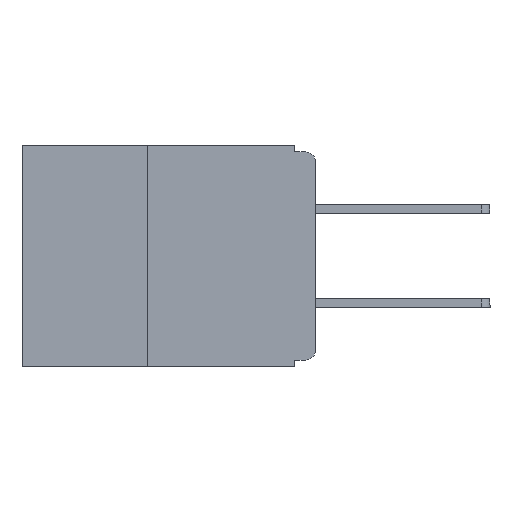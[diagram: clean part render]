
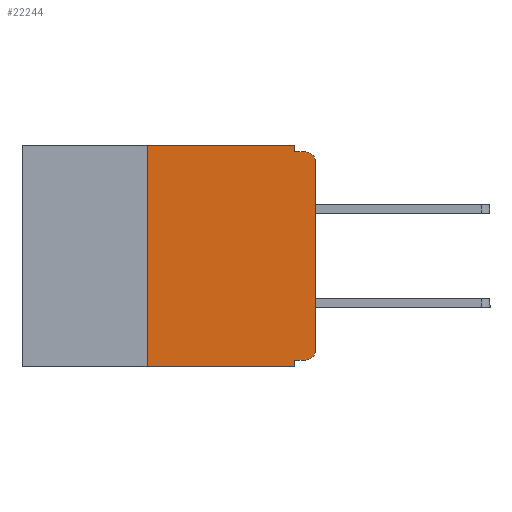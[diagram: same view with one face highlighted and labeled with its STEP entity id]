
A CAD part, left-side view. The second image highlights one B-rep face of the part: STEP entity #22244.
In plain terms, the highlighted planar face has unit normal (-1, 0, 0).
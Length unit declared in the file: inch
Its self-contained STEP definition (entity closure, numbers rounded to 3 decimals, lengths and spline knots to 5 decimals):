
#29 = EDGE_CURVE ( 'NONE', #1006, #13950, #11299, .T. ) ;
#1006 = VERTEX_POINT ( 'NONE', #7758 ) ;
#1195 = VECTOR ( 'NONE', #1696, 39.37008 ) ;
#1295 = CARTESIAN_POINT ( 'NONE',  ( 0., 0.437, 0. ) ) ;
#1696 = DIRECTION ( 'NONE',  ( 0., 1., 0. ) ) ;
#1912 = VERTEX_POINT ( 'NONE', #15409 ) ;
#1956 = ORIENTED_EDGE ( 'NONE', *, *, #19438, .T. ) ;
#3375 = AXIS2_PLACEMENT_3D ( 'NONE', #20729, #7607, #22904 ) ;
#3509 = VECTOR ( 'NONE', #16012, 39.37008 ) ;
#5172 = VECTOR ( 'NONE', #18934, 39.37008 ) ;
#5415 = VERTEX_POINT ( 'NONE', #25262 ) ;
#5727 = VERTEX_POINT ( 'NONE', #28318 ) ;
#6195 = ORIENTED_EDGE ( 'NONE', *, *, #29, .F. ) ;
#6895 = CARTESIAN_POINT ( 'NONE',  ( 0., 0.031, -0.33 ) ) ;
#6993 = VECTOR ( 'NONE', #25163, 39.37008 ) ;
#7089 = CARTESIAN_POINT ( 'NONE',  ( 0., 0.437, -0.33 ) ) ;
#7285 = CARTESIAN_POINT ( 'NONE',  ( 0., 0., -0.01 ) ) ;
#7607 = DIRECTION ( 'NONE',  ( -1., 0., 0. ) ) ;
#7673 = EDGE_CURVE ( 'NONE', #13950, #8500, #27749, .T. ) ;
#7758 = CARTESIAN_POINT ( 'NONE',  ( 0., 0.031, 0. ) ) ;
#7817 = CARTESIAN_POINT ( 'NONE',  ( 0., 0.015, -0.01 ) ) ;
#8166 = ORIENTED_EDGE ( 'NONE', *, *, #11229, .T. ) ;
#8500 = VERTEX_POINT ( 'NONE', #7817 ) ;
#8838 = VERTEX_POINT ( 'NONE', #8943 ) ;
#8943 = CARTESIAN_POINT ( 'NONE',  ( 0., 0., -0.025 ) ) ;
#9079 = ORIENTED_EDGE ( 'NONE', *, *, #23226, .T. ) ;
#9568 = ORIENTED_EDGE ( 'NONE', *, *, #26012, .F. ) ;
#10179 = CARTESIAN_POINT ( 'NONE',  ( 0., 0., 0. ) ) ;
#10299 = DIRECTION ( 'NONE',  ( 0., 0., -1. ) ) ;
#10563 = CIRCLE ( 'NONE', #24649, 0.015 ) ;
#10622 = VECTOR ( 'NONE', #17894, 39.37008 ) ;
#10719 = LINE ( 'NONE', #7089, #16551 ) ;
#11229 = EDGE_CURVE ( 'NONE', #1912, #5415, #12708, .T. ) ;
#11299 = LINE ( 'NONE', #25956, #10622 ) ;
#11710 = CARTESIAN_POINT ( 'NONE',  ( 0., 0.25, -0.33 ) ) ;
#12235 = ORIENTED_EDGE ( 'NONE', *, *, #26722, .F. ) ;
#12324 = CARTESIAN_POINT ( 'NONE',  ( 0., 0.015, -0.025 ) ) ;
#12623 = EDGE_CURVE ( 'NONE', #8838, #8500, #10563, .T. ) ;
#12708 = CIRCLE ( 'NONE', #3375, 0.015 ) ;
#12753 = EDGE_CURVE ( 'NONE', #1912, #5727, #12961, .T. ) ;
#12961 = LINE ( 'NONE', #17100, #1195 ) ;
#13812 = CARTESIAN_POINT ( 'NONE',  ( 0., 0.437, 0. ) ) ;
#13950 = VERTEX_POINT ( 'NONE', #21244 ) ;
#14534 = DIRECTION ( 'NONE',  ( 0., 0., -1. ) ) ;
#14730 = LINE ( 'NONE', #10179, #26298 ) ;
#14974 = EDGE_LOOP ( 'NONE', ( #1956, #27869, #20417, #6195, #9568, #12235, #9079, #20071, #25366, #8166 ) ) ;
#15409 = CARTESIAN_POINT ( 'NONE',  ( 0., 0.015, -0.32 ) ) ;
#16012 = DIRECTION ( 'NONE',  ( 0., -1., 0. ) ) ;
#16551 = VECTOR ( 'NONE', #20289, 39.37008 ) ;
#16734 = CARTESIAN_POINT ( 'NONE',  ( 0., 0.25, -0.33 ) ) ;
#16807 = PLANE ( 'NONE',  #22820 ) ;
#17100 = CARTESIAN_POINT ( 'NONE',  ( 0., 0., -0.32 ) ) ;
#17527 = LINE ( 'NONE', #16734, #5172 ) ;
#17894 = DIRECTION ( 'NONE',  ( 0., 0., -1. ) ) ;
#18116 = DIRECTION ( 'NONE',  ( 0., -1., 0. ) ) ;
#18645 = LINE ( 'NONE', #22978, #6993 ) ;
#18934 = DIRECTION ( 'NONE',  ( 0., 0., 1. ) ) ;
#19438 = EDGE_CURVE ( 'NONE', #5415, #8838, #14730, .T. ) ;
#20071 = ORIENTED_EDGE ( 'NONE', *, *, #22750, .F. ) ;
#20289 = DIRECTION ( 'NONE',  ( 0., -1., 0. ) ) ;
#20417 = ORIENTED_EDGE ( 'NONE', *, *, #7673, .F. ) ;
#20726 = FACE_OUTER_BOUND ( 'NONE', #14974, .T. ) ;
#20729 = CARTESIAN_POINT ( 'NONE',  ( 0., 0.015, -0.305 ) ) ;
#21001 = LINE ( 'NONE', #13812, #3509 ) ;
#21175 = VERTEX_POINT ( 'NONE', #11710 ) ;
#21244 = CARTESIAN_POINT ( 'NONE',  ( 0., 0.031, -0.01 ) ) ;
#21419 = VECTOR ( 'NONE', #18116, 39.37008 ) ;
#22244 = ADVANCED_FACE ( 'NONE', ( #20726 ), #16807, .F. ) ;
#22750 = EDGE_CURVE ( 'NONE', #5727, #26431, #18645, .T. ) ;
#22820 = AXIS2_PLACEMENT_3D ( 'NONE', #1295, #23378, #10299 ) ;
#22904 = DIRECTION ( 'NONE',  ( 0., 0., -1. ) ) ;
#22978 = CARTESIAN_POINT ( 'NONE',  ( 0., 0.031, -0.33 ) ) ;
#23226 = EDGE_CURVE ( 'NONE', #21175, #26431, #10719, .T. ) ;
#23378 = DIRECTION ( 'NONE',  ( 1., 0., 0. ) ) ;
#23645 = VERTEX_POINT ( 'NONE', #27912 ) ;
#24649 = AXIS2_PLACEMENT_3D ( 'NONE', #12324, #27471, #14534 ) ;
#25163 = DIRECTION ( 'NONE',  ( 0., 0., -1. ) ) ;
#25262 = CARTESIAN_POINT ( 'NONE',  ( 0., 0., -0.305 ) ) ;
#25366 = ORIENTED_EDGE ( 'NONE', *, *, #12753, .F. ) ;
#25956 = CARTESIAN_POINT ( 'NONE',  ( 0., 0.031, 0. ) ) ;
#26012 = EDGE_CURVE ( 'NONE', #23645, #1006, #21001, .T. ) ;
#26298 = VECTOR ( 'NONE', #27438, 39.37008 ) ;
#26431 = VERTEX_POINT ( 'NONE', #6895 ) ;
#26722 = EDGE_CURVE ( 'NONE', #21175, #23645, #17527, .T. ) ;
#27438 = DIRECTION ( 'NONE',  ( 0., 0., 1. ) ) ;
#27471 = DIRECTION ( 'NONE',  ( -1., 0., 0. ) ) ;
#27749 = LINE ( 'NONE', #7285, #21419 ) ;
#27869 = ORIENTED_EDGE ( 'NONE', *, *, #12623, .T. ) ;
#27912 = CARTESIAN_POINT ( 'NONE',  ( 0., 0.25, 0. ) ) ;
#28318 = CARTESIAN_POINT ( 'NONE',  ( 0., 0.031, -0.32 ) ) ;
